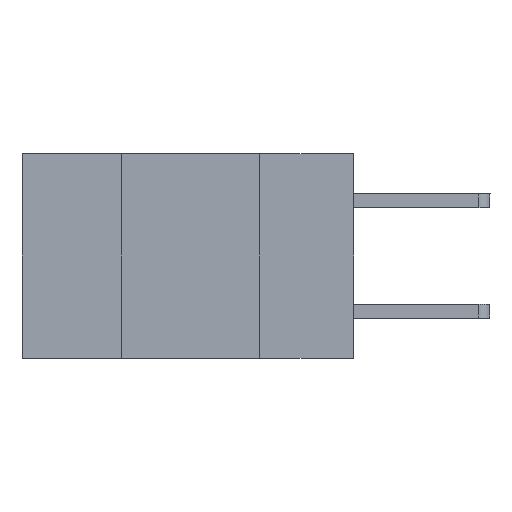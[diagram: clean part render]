
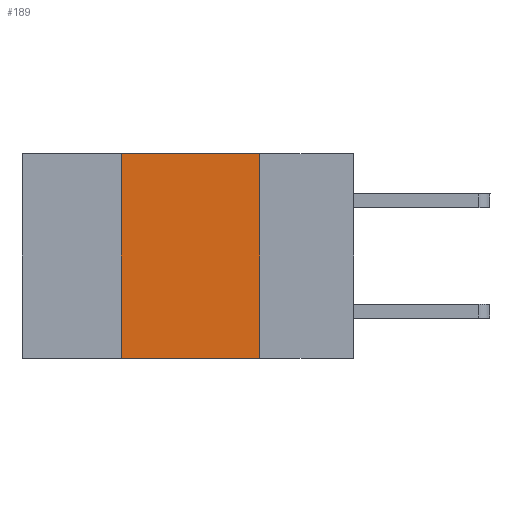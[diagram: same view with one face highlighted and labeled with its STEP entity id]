
A CAD part, left-side view. The second image highlights one B-rep face of the part: STEP entity #189.
In plain terms, the highlighted planar face has unit normal (-1, 0, 0).
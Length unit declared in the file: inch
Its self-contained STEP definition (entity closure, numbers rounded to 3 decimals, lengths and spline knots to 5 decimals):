
#37 = DIRECTION ( 'NONE',  ( 0., -1., 0. ) ) ;
#189 = ADVANCED_FACE ( 'NONE', ( #6594 ), #9693, .F. ) ;
#1233 = CARTESIAN_POINT ( 'NONE',  ( 0., 0.6, 0. ) ) ;
#1553 = CARTESIAN_POINT ( 'NONE',  ( 0., 0.42, -0.37 ) ) ;
#1912 = LINE ( 'NONE', #4703, #10448 ) ;
#2220 = VERTEX_POINT ( 'NONE', #10771 ) ;
#2300 = ORIENTED_EDGE ( 'NONE', *, *, #4536, .T. ) ;
#3022 = LINE ( 'NONE', #10585, #9600 ) ;
#3148 = DIRECTION ( 'NONE',  ( 0., -1., 0. ) ) ;
#3224 = VERTEX_POINT ( 'NONE', #5406 ) ;
#3706 = ORIENTED_EDGE ( 'NONE', *, *, #8127, .F. ) ;
#3979 = ORIENTED_EDGE ( 'NONE', *, *, #11819, .F. ) ;
#4030 = AXIS2_PLACEMENT_3D ( 'NONE', #1233, #5001, #8768 ) ;
#4473 = VERTEX_POINT ( 'NONE', #9131 ) ;
#4536 = EDGE_CURVE ( 'NONE', #8158, #2220, #8696, .T. ) ;
#4703 = CARTESIAN_POINT ( 'NONE',  ( 0., 0.6, 0. ) ) ;
#5001 = DIRECTION ( 'NONE',  ( 1., 0., 0. ) ) ;
#5076 = LINE ( 'NONE', #8336, #12176 ) ;
#5308 = VECTOR ( 'NONE', #37, 39.37008 ) ;
#5406 = CARTESIAN_POINT ( 'NONE',  ( 0., 0.42, 0. ) ) ;
#5428 = DIRECTION ( 'NONE',  ( 0., 0., 1. ) ) ;
#6594 = FACE_OUTER_BOUND ( 'NONE', #10612, .T. ) ;
#8127 = EDGE_CURVE ( 'NONE', #8158, #3224, #5076, .T. ) ;
#8158 = VERTEX_POINT ( 'NONE', #1553 ) ;
#8336 = CARTESIAN_POINT ( 'NONE',  ( 0., 0.42, 0. ) ) ;
#8387 = EDGE_CURVE ( 'NONE', #4473, #2220, #3022, .T. ) ;
#8549 = ORIENTED_EDGE ( 'NONE', *, *, #8387, .F. ) ;
#8632 = CARTESIAN_POINT ( 'NONE',  ( 0., 0.6, -0.37 ) ) ;
#8696 = LINE ( 'NONE', #8632, #5308 ) ;
#8768 = DIRECTION ( 'NONE',  ( 0., 0., -1. ) ) ;
#9131 = CARTESIAN_POINT ( 'NONE',  ( 0., 0.17, 0. ) ) ;
#9600 = VECTOR ( 'NONE', #9634, 39.37008 ) ;
#9634 = DIRECTION ( 'NONE',  ( 0., 0., -1. ) ) ;
#9693 = PLANE ( 'NONE',  #4030 ) ;
#10448 = VECTOR ( 'NONE', #3148, 39.37008 ) ;
#10585 = CARTESIAN_POINT ( 'NONE',  ( 0., 0.17, 0. ) ) ;
#10612 = EDGE_LOOP ( 'NONE', ( #8549, #3979, #3706, #2300 ) ) ;
#10771 = CARTESIAN_POINT ( 'NONE',  ( 0., 0.17, -0.37 ) ) ;
#11819 = EDGE_CURVE ( 'NONE', #3224, #4473, #1912, .T. ) ;
#12176 = VECTOR ( 'NONE', #5428, 39.37008 ) ;
